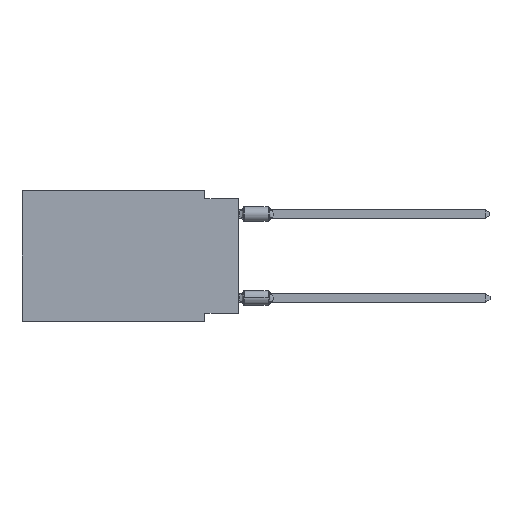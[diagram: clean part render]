
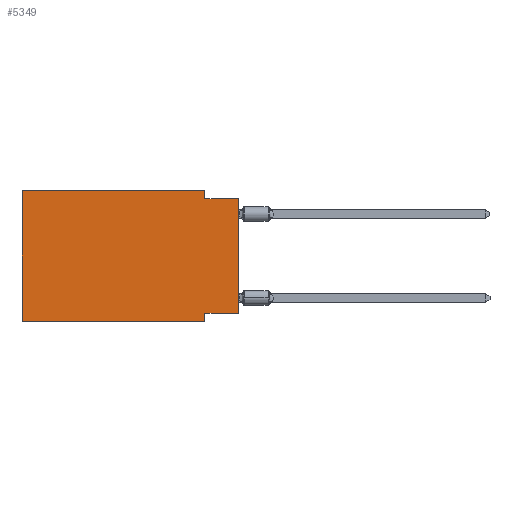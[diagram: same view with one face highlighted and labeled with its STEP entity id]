
A CAD part, left-side view. The second image highlights one B-rep face of the part: STEP entity #5349.
In plain terms, the highlighted planar face has unit normal (-1, 0, 0).
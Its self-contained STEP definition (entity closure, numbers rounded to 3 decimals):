
#134 = CARTESIAN_POINT ( 'NONE',  ( 0., 2.54, -9.906 ) ) ;
#344 = DIRECTION ( 'NONE',  ( 0., 0., -1. ) ) ;
#554 = DIRECTION ( 'NONE',  ( 0., -1., 0. ) ) ;
#647 = ORIENTED_EDGE ( 'NONE', *, *, #7394, .F. ) ;
#925 = LINE ( 'NONE', #9698, #1130 ) ;
#1130 = VECTOR ( 'NONE', #16467, 1000. ) ;
#2132 = CARTESIAN_POINT ( 'NONE',  ( 0., 2.54, 0. ) ) ;
#2203 = CARTESIAN_POINT ( 'NONE',  ( 0., 2.54, -0.635 ) ) ;
#3171 = ORIENTED_EDGE ( 'NONE', *, *, #21554, .F. ) ;
#3580 = VERTEX_POINT ( 'NONE', #6808 ) ;
#3764 = LINE ( 'NONE', #14857, #23281 ) ;
#4049 = EDGE_CURVE ( 'NONE', #14262, #23508, #24550, .T. ) ;
#4217 = ORIENTED_EDGE ( 'NONE', *, *, #5235, .F. ) ;
#4936 = EDGE_LOOP ( 'NONE', ( #12073, #23207, #647, #27652, #3171, #20871, #16320, #4217 ) ) ;
#5235 = EDGE_CURVE ( 'NONE', #3580, #18186, #3764, .T. ) ;
#5349 = ADVANCED_FACE ( 'NONE', ( #17860 ), #6214, .F. ) ;
#5659 = LINE ( 'NONE', #23618, #9341 ) ;
#6214 = PLANE ( 'NONE',  #28296 ) ;
#6553 = VERTEX_POINT ( 'NONE', #2203 ) ;
#6808 = CARTESIAN_POINT ( 'NONE',  ( 0., 0., -9.271 ) ) ;
#7322 = VERTEX_POINT ( 'NONE', #13080 ) ;
#7394 = EDGE_CURVE ( 'NONE', #7322, #6553, #19805, .T. ) ;
#8657 = DIRECTION ( 'NONE',  ( 0., -1., 0. ) ) ;
#9190 = CARTESIAN_POINT ( 'NONE',  ( 0., 16.383, -9.906 ) ) ;
#9341 = VECTOR ( 'NONE', #12737, 1000. ) ;
#9458 = VECTOR ( 'NONE', #554, 1000. ) ;
#9698 = CARTESIAN_POINT ( 'NONE',  ( 0., 16.383, 0. ) ) ;
#10834 = VECTOR ( 'NONE', #23900, 1000. ) ;
#12073 = ORIENTED_EDGE ( 'NONE', *, *, #12992, .T. ) ;
#12717 = DIRECTION ( 'NONE',  ( 0., 1., 0. ) ) ;
#12737 = DIRECTION ( 'NONE',  ( 0., 0., 1. ) ) ;
#12992 = EDGE_CURVE ( 'NONE', #3580, #14924, #5659, .T. ) ;
#13062 = CARTESIAN_POINT ( 'NONE',  ( 0., 2.54, -9.271 ) ) ;
#13080 = CARTESIAN_POINT ( 'NONE',  ( 0., 2.54, 0. ) ) ;
#13097 = EDGE_CURVE ( 'NONE', #18186, #23508, #15032, .T. ) ;
#13271 = CARTESIAN_POINT ( 'NONE',  ( 0., 0., -0.635 ) ) ;
#13399 = LINE ( 'NONE', #13271, #19042 ) ;
#14262 = VERTEX_POINT ( 'NONE', #19608 ) ;
#14857 = CARTESIAN_POINT ( 'NONE',  ( 0., 0., -9.271 ) ) ;
#14924 = VERTEX_POINT ( 'NONE', #19104 ) ;
#15032 = LINE ( 'NONE', #23769, #16888 ) ;
#15175 = CARTESIAN_POINT ( 'NONE',  ( 0., 16.383, 0. ) ) ;
#15436 = DIRECTION ( 'NONE',  ( 1., 0., 0. ) ) ;
#15708 = EDGE_CURVE ( 'NONE', #24246, #7322, #925, .T. ) ;
#16320 = ORIENTED_EDGE ( 'NONE', *, *, #13097, .F. ) ;
#16390 = EDGE_CURVE ( 'NONE', #6553, #14924, #13399, .T. ) ;
#16467 = DIRECTION ( 'NONE',  ( 0., -1., 0. ) ) ;
#16888 = VECTOR ( 'NONE', #344, 1000. ) ;
#17860 = FACE_OUTER_BOUND ( 'NONE', #4936, .T. ) ;
#18186 = VERTEX_POINT ( 'NONE', #13062 ) ;
#19042 = VECTOR ( 'NONE', #8657, 1000. ) ;
#19104 = CARTESIAN_POINT ( 'NONE',  ( 0., 0., -0.635 ) ) ;
#19608 = CARTESIAN_POINT ( 'NONE',  ( 0., 16.383, -9.906 ) ) ;
#19805 = LINE ( 'NONE', #2132, #28191 ) ;
#20184 = LINE ( 'NONE', #15175, #10834 ) ;
#20871 = ORIENTED_EDGE ( 'NONE', *, *, #4049, .T. ) ;
#21554 = EDGE_CURVE ( 'NONE', #14262, #24246, #20184, .T. ) ;
#21604 = DIRECTION ( 'NONE',  ( 0., 0., -1. ) ) ;
#22029 = CARTESIAN_POINT ( 'NONE',  ( 0., 16.383, 0. ) ) ;
#23207 = ORIENTED_EDGE ( 'NONE', *, *, #16390, .F. ) ;
#23281 = VECTOR ( 'NONE', #12717, 1000. ) ;
#23508 = VERTEX_POINT ( 'NONE', #134 ) ;
#23618 = CARTESIAN_POINT ( 'NONE',  ( 0., 0., 0. ) ) ;
#23769 = CARTESIAN_POINT ( 'NONE',  ( 0., 2.54, -9.906 ) ) ;
#23900 = DIRECTION ( 'NONE',  ( 0., 0., 1. ) ) ;
#24246 = VERTEX_POINT ( 'NONE', #22029 ) ;
#24550 = LINE ( 'NONE', #9190, #9458 ) ;
#26156 = CARTESIAN_POINT ( 'NONE',  ( 0., 16.383, 0. ) ) ;
#27652 = ORIENTED_EDGE ( 'NONE', *, *, #15708, .F. ) ;
#27980 = DIRECTION ( 'NONE',  ( 0., 0., -1. ) ) ;
#28191 = VECTOR ( 'NONE', #27980, 1000. ) ;
#28296 = AXIS2_PLACEMENT_3D ( 'NONE', #26156, #15436, #21604 ) ;
